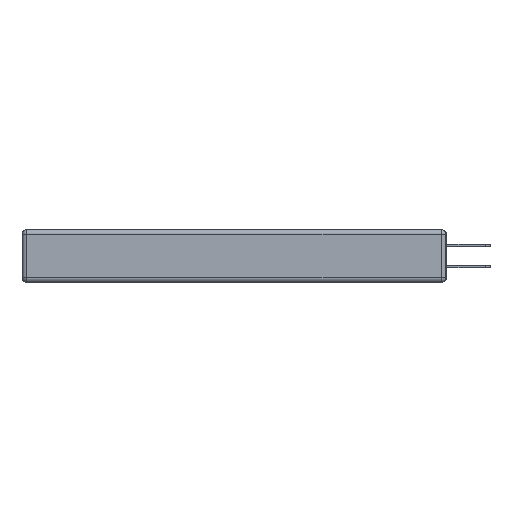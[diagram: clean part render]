
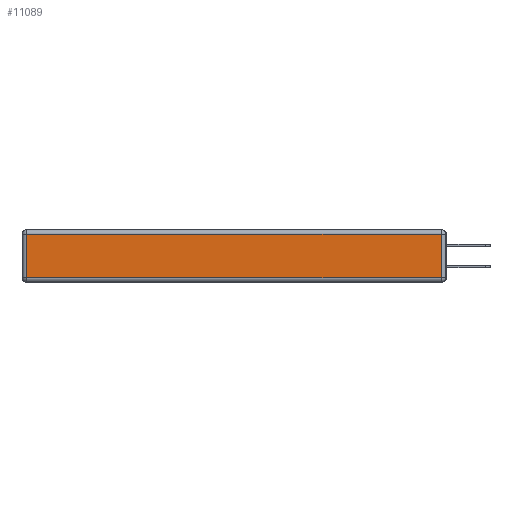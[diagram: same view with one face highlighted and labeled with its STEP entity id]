
A CAD part, left-side view. The second image highlights one B-rep face of the part: STEP entity #11089.
In plain terms, the highlighted planar face has unit normal (-1, 0, 0).
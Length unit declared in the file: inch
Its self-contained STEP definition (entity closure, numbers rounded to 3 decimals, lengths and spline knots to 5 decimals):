
#306 = VECTOR ( 'NONE', #19817, 39.37008 ) ;
#763 = CARTESIAN_POINT ( 'NONE',  ( 0., 2.72, -0.343 ) ) ;
#1143 = CARTESIAN_POINT ( 'NONE',  ( 0., 0.03, -0.03 ) ) ;
#1905 = CARTESIAN_POINT ( 'NONE',  ( 0., 2.72, -0.03 ) ) ;
#2112 = DIRECTION ( 'NONE',  ( -1., 0., 0. ) ) ;
#2292 = PLANE ( 'NONE',  #4555 ) ;
#4555 = AXIS2_PLACEMENT_3D ( 'NONE', #10466, #2112, #8562 ) ;
#5058 = CARTESIAN_POINT ( 'NONE',  ( 0., 0., -0.313 ) ) ;
#5525 = ORIENTED_EDGE ( 'NONE', *, *, #9355, .T. ) ;
#5790 = VERTEX_POINT ( 'NONE', #1905 ) ;
#6208 = VECTOR ( 'NONE', #25882, 39.37008 ) ;
#7977 = VERTEX_POINT ( 'NONE', #24756 ) ;
#8562 = DIRECTION ( 'NONE',  ( 0., 0., 1. ) ) ;
#8686 = EDGE_CURVE ( 'NONE', #25591, #5790, #13102, .T. ) ;
#8990 = DIRECTION ( 'NONE',  ( 0., 0., -1. ) ) ;
#9355 = EDGE_CURVE ( 'NONE', #7977, #20181, #15655, .T. ) ;
#9409 = CARTESIAN_POINT ( 'NONE',  ( 0., 0.03, -0.313 ) ) ;
#9645 = CARTESIAN_POINT ( 'NONE',  ( 0., 0.03, -0.343 ) ) ;
#10079 = LINE ( 'NONE', #9645, #21461 ) ;
#10466 = CARTESIAN_POINT ( 'NONE',  ( 0., 0., -0.343 ) ) ;
#11088 = LINE ( 'NONE', #763, #27056 ) ;
#11089 = ADVANCED_FACE ( 'NONE', ( #21836 ), #2292, .T. ) ;
#11726 = EDGE_CURVE ( 'NONE', #20181, #25591, #10079, .T. ) ;
#13102 = LINE ( 'NONE', #16074, #306 ) ;
#14387 = ORIENTED_EDGE ( 'NONE', *, *, #20845, .T. ) ;
#15155 = EDGE_LOOP ( 'NONE', ( #5525, #18665, #24408, #14387 ) ) ;
#15655 = LINE ( 'NONE', #5058, #6208 ) ;
#16074 = CARTESIAN_POINT ( 'NONE',  ( 0., 2.75, -0.03 ) ) ;
#18665 = ORIENTED_EDGE ( 'NONE', *, *, #11726, .T. ) ;
#19817 = DIRECTION ( 'NONE',  ( 0., 1., 0. ) ) ;
#20181 = VERTEX_POINT ( 'NONE', #9409 ) ;
#20845 = EDGE_CURVE ( 'NONE', #5790, #7977, #11088, .T. ) ;
#21461 = VECTOR ( 'NONE', #24177, 39.37008 ) ;
#21836 = FACE_OUTER_BOUND ( 'NONE', #15155, .T. ) ;
#24177 = DIRECTION ( 'NONE',  ( 0., 0., 1. ) ) ;
#24408 = ORIENTED_EDGE ( 'NONE', *, *, #8686, .T. ) ;
#24756 = CARTESIAN_POINT ( 'NONE',  ( 0., 2.72, -0.313 ) ) ;
#25591 = VERTEX_POINT ( 'NONE', #1143 ) ;
#25882 = DIRECTION ( 'NONE',  ( 0., -1., 0. ) ) ;
#27056 = VECTOR ( 'NONE', #8990, 39.37008 ) ;
